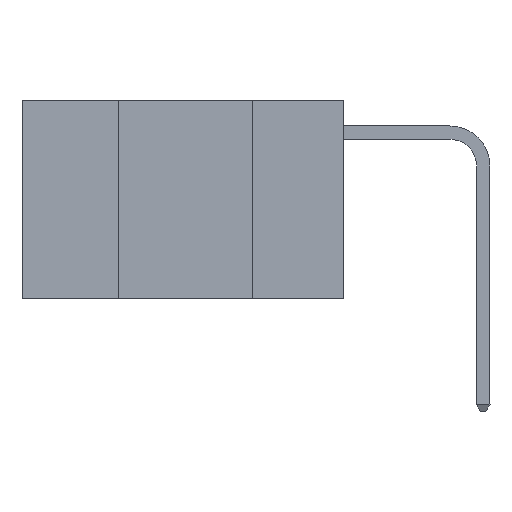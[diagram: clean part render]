
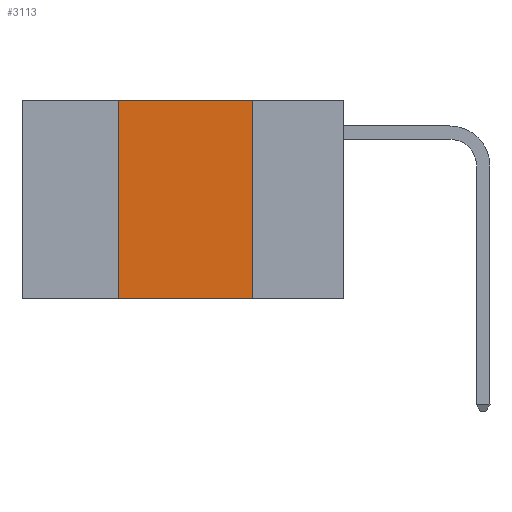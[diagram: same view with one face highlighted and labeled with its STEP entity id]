
A CAD part, left-side view. The second image highlights one B-rep face of the part: STEP entity #3113.
In plain terms, the highlighted planar face has unit normal (-1, 0, 0).
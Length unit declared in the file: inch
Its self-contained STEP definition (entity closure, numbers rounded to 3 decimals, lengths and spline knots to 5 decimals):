
#110 = ORIENTED_EDGE ( 'NONE', *, *, #13931, .F. ) ;
#363 = VERTEX_POINT ( 'NONE', #15277 ) ;
#372 = FACE_OUTER_BOUND ( 'NONE', #8754, .T. ) ;
#868 = DIRECTION ( 'NONE',  ( 0., 0., -1. ) ) ;
#1131 = EDGE_CURVE ( 'NONE', #1903, #14439, #16218, .T. ) ;
#1632 = VECTOR ( 'NONE', #868, 39.37008 ) ;
#1903 = VERTEX_POINT ( 'NONE', #5939 ) ;
#1958 = DIRECTION ( 'NONE',  ( 0., -1., 0. ) ) ;
#2413 = LINE ( 'NONE', #15245, #1632 ) ;
#2612 = CARTESIAN_POINT ( 'NONE',  ( 0., 0.17, 0. ) ) ;
#2857 = DIRECTION ( 'NONE',  ( 1., 0., 0. ) ) ;
#2958 = CARTESIAN_POINT ( 'NONE',  ( 0., 0.42, 0. ) ) ;
#3113 = ADVANCED_FACE ( 'NONE', ( #372 ), #12047, .F. ) ;
#3800 = ORIENTED_EDGE ( 'NONE', *, *, #12434, .F. ) ;
#4166 = CARTESIAN_POINT ( 'NONE',  ( 0., 0.6, -0.37 ) ) ;
#5514 = VERTEX_POINT ( 'NONE', #2612 ) ;
#5621 = DIRECTION ( 'NONE',  ( 0., 0., -1. ) ) ;
#5723 = ORIENTED_EDGE ( 'NONE', *, *, #7353, .F. ) ;
#5853 = CARTESIAN_POINT ( 'NONE',  ( 0., 0.6, 0. ) ) ;
#5939 = CARTESIAN_POINT ( 'NONE',  ( 0., 0.42, -0.37 ) ) ;
#6919 = CARTESIAN_POINT ( 'NONE',  ( 0., 0.6, 0. ) ) ;
#7353 = EDGE_CURVE ( 'NONE', #363, #5514, #12184, .T. ) ;
#8199 = DIRECTION ( 'NONE',  ( 0., 0., 1. ) ) ;
#8359 = AXIS2_PLACEMENT_3D ( 'NONE', #6919, #2857, #5621 ) ;
#8713 = VECTOR ( 'NONE', #9441, 39.37008 ) ;
#8754 = EDGE_LOOP ( 'NONE', ( #110, #5723, #3800, #15567 ) ) ;
#9441 = DIRECTION ( 'NONE',  ( 0., -1., 0. ) ) ;
#12047 = PLANE ( 'NONE',  #8359 ) ;
#12184 = LINE ( 'NONE', #5853, #16345 ) ;
#12434 = EDGE_CURVE ( 'NONE', #1903, #363, #14749, .T. ) ;
#13517 = CARTESIAN_POINT ( 'NONE',  ( 0., 0.17, -0.37 ) ) ;
#13931 = EDGE_CURVE ( 'NONE', #5514, #14439, #2413, .T. ) ;
#14439 = VERTEX_POINT ( 'NONE', #13517 ) ;
#14749 = LINE ( 'NONE', #2958, #15318 ) ;
#15245 = CARTESIAN_POINT ( 'NONE',  ( 0., 0.17, 0. ) ) ;
#15277 = CARTESIAN_POINT ( 'NONE',  ( 0., 0.42, 0. ) ) ;
#15318 = VECTOR ( 'NONE', #8199, 39.37008 ) ;
#15567 = ORIENTED_EDGE ( 'NONE', *, *, #1131, .T. ) ;
#16218 = LINE ( 'NONE', #4166, #8713 ) ;
#16345 = VECTOR ( 'NONE', #1958, 39.37008 ) ;
